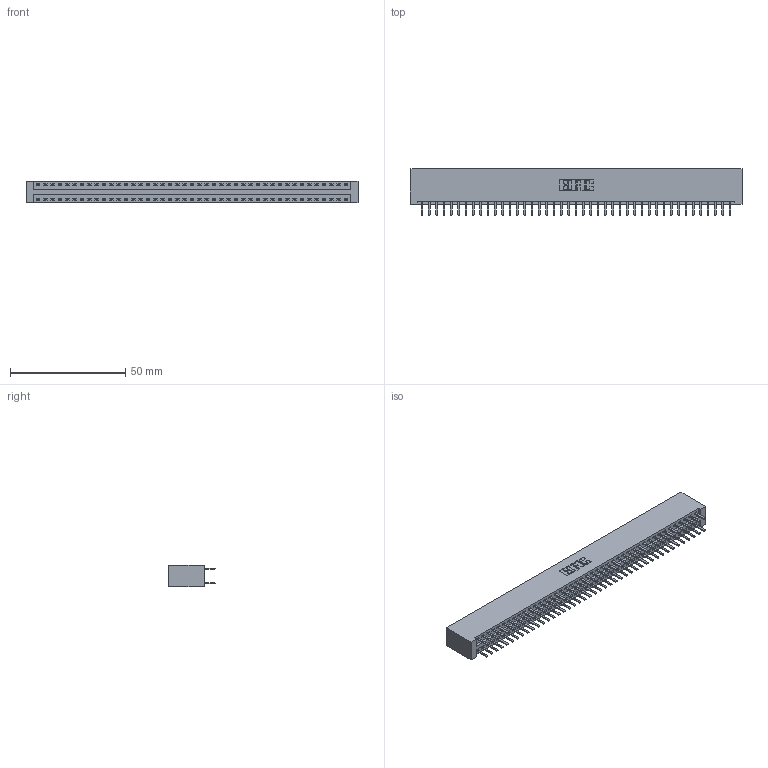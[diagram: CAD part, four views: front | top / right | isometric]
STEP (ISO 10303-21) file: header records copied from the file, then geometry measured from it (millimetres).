
FILE_DESCRIPTION (( 'STEP AP203' ), '1' );
FILE_NAME ('396-086-520-201.STEP', '2018-09-10T02:27:18', ( '' ), ( '' ), 'SwSTEP 2.0', 'SolidWorks 2016', '' );
FILE_SCHEMA (( 'CONFIG_CONTROL_DESIGN' ));
Length unit declared in the file: inch
Products named in the file (3): 346 Part_No Mounting Lugs; 345-292-001_345-293-120; 396-086-520-201
Assembly tree (87 placements, depth 2):
  396-086-520-201
    346 Part_No Mounting Lugs
    345-292-001_345-293-120  x86
Bounding box: 143.76 x 20.02 x 9.4 mm (x, y, z)
Volume: 14562 mm3; surface area: 20106.8 mm2
Topology: 87 solids, 87 shells, 4930 faces, 14323 edges, 9318 vertices
Faces by surface type: plane 3254, cylinder 1676
Entity records: 27765 total; most frequent: CARTESIAN_POINT 4584, ORIENTED_EDGE 4506, DIRECTION 4073, EDGE_CURVE 2253, VECTOR 1953, LINE 1953, VERTEX_POINT 1498, AXIS2_PLACEMENT_3D 1060
